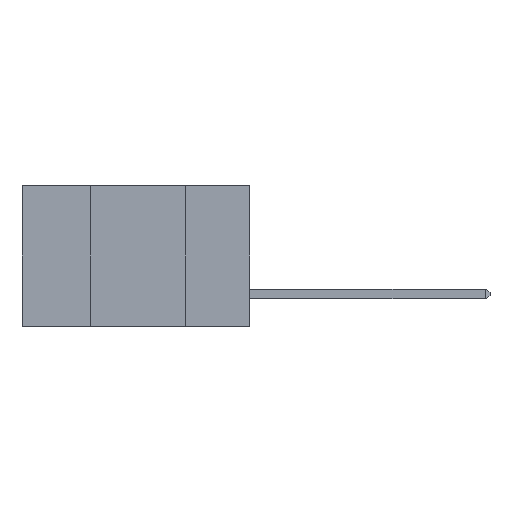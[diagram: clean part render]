
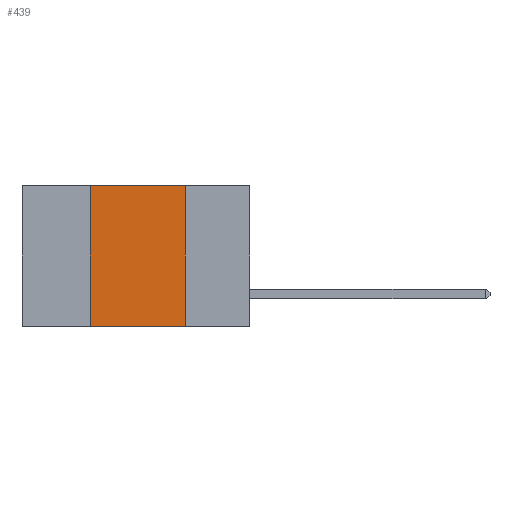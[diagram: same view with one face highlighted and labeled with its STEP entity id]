
A CAD part, left-side view. The second image highlights one B-rep face of the part: STEP entity #439.
In plain terms, the highlighted planar face has unit normal (-1, 0, 0).
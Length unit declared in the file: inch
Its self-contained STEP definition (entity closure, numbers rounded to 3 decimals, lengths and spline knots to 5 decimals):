
#206 = VERTEX_POINT ( 'NONE', #11625 ) ;
#384 = LINE ( 'NONE', #1169, #2731 ) ;
#439 = ADVANCED_FACE ( 'NONE', ( #700 ), #8143, .F. ) ;
#518 = CARTESIAN_POINT ( 'NONE',  ( 0., 0.42, -0.37 ) ) ;
#700 = FACE_OUTER_BOUND ( 'NONE', #8291, .T. ) ;
#837 = DIRECTION ( 'NONE',  ( 1., 0., 0. ) ) ;
#933 = CARTESIAN_POINT ( 'NONE',  ( 0., 0.6, 0. ) ) ;
#1009 = VERTEX_POINT ( 'NONE', #5679 ) ;
#1116 = ORIENTED_EDGE ( 'NONE', *, *, #1632, .F. ) ;
#1169 = CARTESIAN_POINT ( 'NONE',  ( 0., 0.6, 0. ) ) ;
#1205 = CARTESIAN_POINT ( 'NONE',  ( 0., 0.42, 0. ) ) ;
#1271 = CARTESIAN_POINT ( 'NONE',  ( 0., 0.17, 0. ) ) ;
#1630 = VERTEX_POINT ( 'NONE', #518 ) ;
#1632 = EDGE_CURVE ( 'NONE', #10261, #1009, #384, .T. ) ;
#1751 = LINE ( 'NONE', #1205, #6710 ) ;
#1803 = DIRECTION ( 'NONE',  ( 0., 0., -1. ) ) ;
#2282 = DIRECTION ( 'NONE',  ( 0., 0., -1. ) ) ;
#2358 = ORIENTED_EDGE ( 'NONE', *, *, #6799, .T. ) ;
#2731 = VECTOR ( 'NONE', #4817, 39.37008 ) ;
#3729 = EDGE_CURVE ( 'NONE', #1630, #10261, #1751, .T. ) ;
#4016 = VECTOR ( 'NONE', #7845, 39.37008 ) ;
#4671 = ORIENTED_EDGE ( 'NONE', *, *, #9547, .F. ) ;
#4817 = DIRECTION ( 'NONE',  ( 0., -1., 0. ) ) ;
#5230 = ORIENTED_EDGE ( 'NONE', *, *, #3729, .F. ) ;
#5558 = CARTESIAN_POINT ( 'NONE',  ( 0., 0.42, 0. ) ) ;
#5679 = CARTESIAN_POINT ( 'NONE',  ( 0., 0.17, 0. ) ) ;
#6167 = DIRECTION ( 'NONE',  ( 0., 0., 1. ) ) ;
#6710 = VECTOR ( 'NONE', #6167, 39.37008 ) ;
#6799 = EDGE_CURVE ( 'NONE', #1630, #206, #9182, .T. ) ;
#7845 = DIRECTION ( 'NONE',  ( 0., -1., 0. ) ) ;
#8143 = PLANE ( 'NONE',  #12253 ) ;
#8291 = EDGE_LOOP ( 'NONE', ( #4671, #1116, #5230, #2358 ) ) ;
#9182 = LINE ( 'NONE', #9386, #4016 ) ;
#9386 = CARTESIAN_POINT ( 'NONE',  ( 0., 0.6, -0.37 ) ) ;
#9547 = EDGE_CURVE ( 'NONE', #1009, #206, #11737, .T. ) ;
#10261 = VERTEX_POINT ( 'NONE', #5558 ) ;
#11466 = VECTOR ( 'NONE', #2282, 39.37008 ) ;
#11625 = CARTESIAN_POINT ( 'NONE',  ( 0., 0.17, -0.37 ) ) ;
#11737 = LINE ( 'NONE', #1271, #11466 ) ;
#12253 = AXIS2_PLACEMENT_3D ( 'NONE', #933, #837, #1803 ) ;
